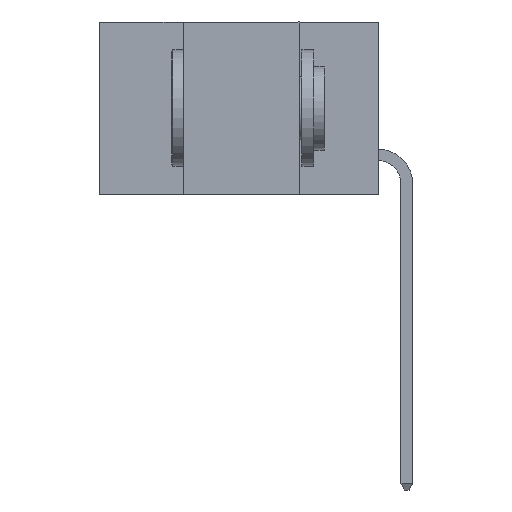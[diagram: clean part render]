
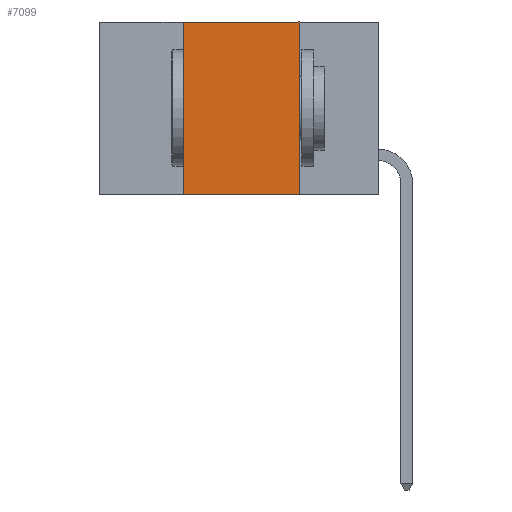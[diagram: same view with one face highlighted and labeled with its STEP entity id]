
A CAD part, left-side view. The second image highlights one B-rep face of the part: STEP entity #7099.
In plain terms, the highlighted planar face has unit normal (-1, 0, 0).
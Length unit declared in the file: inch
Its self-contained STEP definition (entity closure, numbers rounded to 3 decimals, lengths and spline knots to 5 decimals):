
#155 = VERTEX_POINT ( 'NONE', #7173 ) ;
#1206 = EDGE_CURVE ( 'NONE', #4564, #155, #5395, .T. ) ;
#1265 = CARTESIAN_POINT ( 'NONE',  ( 0., 0.6, -0.37 ) ) ;
#1474 = CARTESIAN_POINT ( 'NONE',  ( 0., 0.6, 0. ) ) ;
#2107 = DIRECTION ( 'NONE',  ( 0., -1., 0. ) ) ;
#2298 = EDGE_CURVE ( 'NONE', #4564, #12471, #6377, .T. ) ;
#3213 = ORIENTED_EDGE ( 'NONE', *, *, #5411, .F. ) ;
#3347 = EDGE_CURVE ( 'NONE', #12471, #19523, #19053, .T. ) ;
#3618 = ORIENTED_EDGE ( 'NONE', *, *, #3347, .F. ) ;
#3638 = ORIENTED_EDGE ( 'NONE', *, *, #2298, .F. ) ;
#3808 = ORIENTED_EDGE ( 'NONE', *, *, #1206, .T. ) ;
#4295 = VECTOR ( 'NONE', #10474, 39.37008 ) ;
#4564 = VERTEX_POINT ( 'NONE', #10653 ) ;
#5395 = LINE ( 'NONE', #1265, #9187 ) ;
#5411 = EDGE_CURVE ( 'NONE', #19523, #155, #8572, .T. ) ;
#5971 = FACE_OUTER_BOUND ( 'NONE', #14758, .T. ) ;
#6044 = AXIS2_PLACEMENT_3D ( 'NONE', #19953, #14062, #14045 ) ;
#6377 = LINE ( 'NONE', #16710, #10201 ) ;
#7099 = ADVANCED_FACE ( 'NONE', ( #5971 ), #15055, .F. ) ;
#7173 = CARTESIAN_POINT ( 'NONE',  ( 0., 0.17, -0.37 ) ) ;
#8572 = LINE ( 'NONE', #9196, #4295 ) ;
#9187 = VECTOR ( 'NONE', #13379, 39.37008 ) ;
#9196 = CARTESIAN_POINT ( 'NONE',  ( 0., 0.17, -0.37 ) ) ;
#10201 = VECTOR ( 'NONE', #16671, 39.37008 ) ;
#10474 = DIRECTION ( 'NONE',  ( 0., 0., -1. ) ) ;
#10653 = CARTESIAN_POINT ( 'NONE',  ( 0., 0.42, -0.37 ) ) ;
#11419 = VECTOR ( 'NONE', #2107, 39.37008 ) ;
#12471 = VERTEX_POINT ( 'NONE', #15590 ) ;
#13379 = DIRECTION ( 'NONE',  ( 0., -1., 0. ) ) ;
#14045 = DIRECTION ( 'NONE',  ( 0., 0., -1. ) ) ;
#14062 = DIRECTION ( 'NONE',  ( 1., 0., 0. ) ) ;
#14758 = EDGE_LOOP ( 'NONE', ( #3213, #3618, #3638, #3808 ) ) ;
#15055 = PLANE ( 'NONE',  #6044 ) ;
#15590 = CARTESIAN_POINT ( 'NONE',  ( 0., 0.42, 0. ) ) ;
#16671 = DIRECTION ( 'NONE',  ( 0., 0., 1. ) ) ;
#16710 = CARTESIAN_POINT ( 'NONE',  ( 0., 0.42, -0.37 ) ) ;
#19053 = LINE ( 'NONE', #1474, #11419 ) ;
#19523 = VERTEX_POINT ( 'NONE', #20042 ) ;
#19953 = CARTESIAN_POINT ( 'NONE',  ( 0., 0.6, 0. ) ) ;
#20042 = CARTESIAN_POINT ( 'NONE',  ( 0., 0.17, 0. ) ) ;
